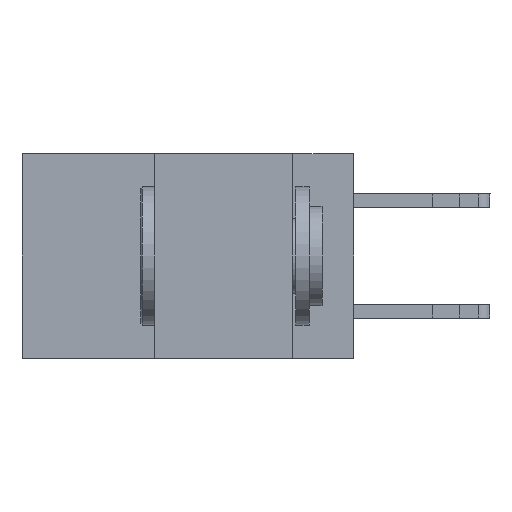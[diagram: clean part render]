
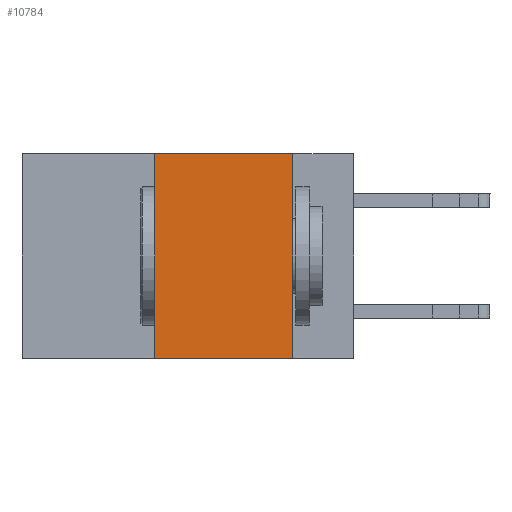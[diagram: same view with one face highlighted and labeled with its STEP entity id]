
A CAD part, left-side view. The second image highlights one B-rep face of the part: STEP entity #10784.
In plain terms, the highlighted planar face has unit normal (-1, 0, 0).
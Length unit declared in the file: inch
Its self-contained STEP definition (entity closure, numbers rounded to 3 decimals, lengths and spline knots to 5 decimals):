
#1207 = VECTOR ( 'NONE', #22893, 39.37008 ) ;
#1556 = CARTESIAN_POINT ( 'NONE',  ( 0., 0.36, 0. ) ) ;
#3035 = EDGE_LOOP ( 'NONE', ( #11430, #8628, #11030, #17161 ) ) ;
#3348 = EDGE_CURVE ( 'NONE', #13504, #13965, #14988, .T. ) ;
#4083 = LINE ( 'NONE', #17874, #6326 ) ;
#4913 = DIRECTION ( 'NONE',  ( 0., 0., -1. ) ) ;
#6326 = VECTOR ( 'NONE', #17985, 39.37008 ) ;
#6617 = CARTESIAN_POINT ( 'NONE',  ( 0., 0.36, -0.37 ) ) ;
#6887 = CARTESIAN_POINT ( 'NONE',  ( 0., 0.6, 0. ) ) ;
#8127 = VECTOR ( 'NONE', #10066, 39.37008 ) ;
#8172 = EDGE_CURVE ( 'NONE', #14403, #12987, #8665, .T. ) ;
#8554 = LINE ( 'NONE', #15688, #1207 ) ;
#8628 = ORIENTED_EDGE ( 'NONE', *, *, #3348, .F. ) ;
#8665 = LINE ( 'NONE', #15813, #15313 ) ;
#10066 = DIRECTION ( 'NONE',  ( 0., -1., 0. ) ) ;
#10650 = DIRECTION ( 'NONE',  ( 1., 0., 0. ) ) ;
#10784 = ADVANCED_FACE ( 'NONE', ( #23121 ), #19604, .F. ) ;
#11030 = ORIENTED_EDGE ( 'NONE', *, *, #13232, .F. ) ;
#11430 = ORIENTED_EDGE ( 'NONE', *, *, #13974, .F. ) ;
#12987 = VERTEX_POINT ( 'NONE', #14136 ) ;
#13232 = EDGE_CURVE ( 'NONE', #14403, #13504, #4083, .T. ) ;
#13504 = VERTEX_POINT ( 'NONE', #1556 ) ;
#13965 = VERTEX_POINT ( 'NONE', #21012 ) ;
#13974 = EDGE_CURVE ( 'NONE', #13965, #12987, #8554, .T. ) ;
#14136 = CARTESIAN_POINT ( 'NONE',  ( 0., 0.11, -0.37 ) ) ;
#14403 = VERTEX_POINT ( 'NONE', #6617 ) ;
#14988 = LINE ( 'NONE', #19001, #8127 ) ;
#15313 = VECTOR ( 'NONE', #23013, 39.37008 ) ;
#15688 = CARTESIAN_POINT ( 'NONE',  ( 0., 0.11, 0. ) ) ;
#15813 = CARTESIAN_POINT ( 'NONE',  ( 0., 0.6, -0.37 ) ) ;
#17161 = ORIENTED_EDGE ( 'NONE', *, *, #8172, .T. ) ;
#17874 = CARTESIAN_POINT ( 'NONE',  ( 0., 0.36, 0. ) ) ;
#17985 = DIRECTION ( 'NONE',  ( 0., 0., 1. ) ) ;
#19001 = CARTESIAN_POINT ( 'NONE',  ( 0., 0.6, 0. ) ) ;
#19604 = PLANE ( 'NONE',  #20616 ) ;
#20616 = AXIS2_PLACEMENT_3D ( 'NONE', #6887, #10650, #4913 ) ;
#21012 = CARTESIAN_POINT ( 'NONE',  ( 0., 0.11, 0. ) ) ;
#22893 = DIRECTION ( 'NONE',  ( 0., 0., -1. ) ) ;
#23013 = DIRECTION ( 'NONE',  ( 0., -1., 0. ) ) ;
#23121 = FACE_OUTER_BOUND ( 'NONE', #3035, .T. ) ;
